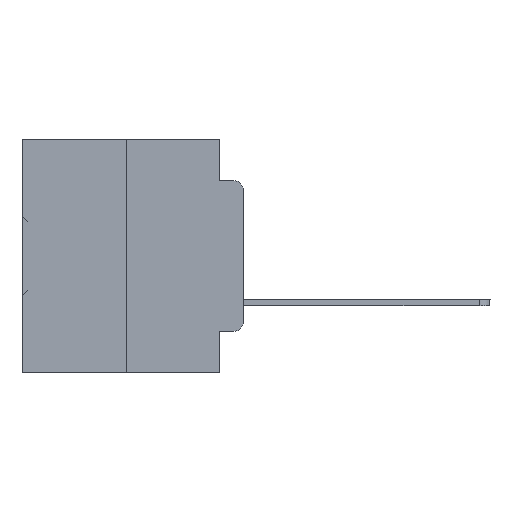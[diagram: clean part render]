
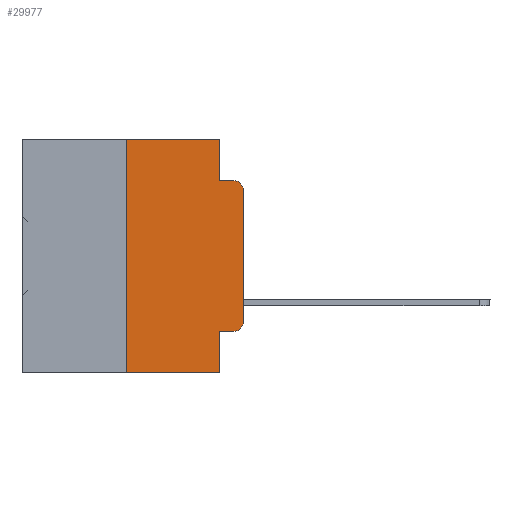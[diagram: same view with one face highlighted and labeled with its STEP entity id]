
A CAD part, left-side view. The second image highlights one B-rep face of the part: STEP entity #29977.
In plain terms, the highlighted planar face has unit normal (-1, 0, 0).
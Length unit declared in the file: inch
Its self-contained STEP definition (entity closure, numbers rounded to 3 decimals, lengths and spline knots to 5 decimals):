
#377 = VERTEX_POINT ( 'NONE', #6065 ) ;
#1059 = AXIS2_PLACEMENT_3D ( 'NONE', #21264, #10166, #18961 ) ;
#1066 = VECTOR ( 'NONE', #21905, 39.37008 ) ;
#1268 = EDGE_CURVE ( 'NONE', #36753, #8072, #4302, .T. ) ;
#1319 = CIRCLE ( 'NONE', #37366, 0.02 ) ;
#1784 = EDGE_CURVE ( 'NONE', #7292, #15828, #33051, .T. ) ;
#2065 = ORIENTED_EDGE ( 'NONE', *, *, #7020, .F. ) ;
#2233 = CARTESIAN_POINT ( 'NONE',  ( 0., 0.051, -0.4115 ) ) ;
#2725 = CARTESIAN_POINT ( 'NONE',  ( 0., 0.051, -0.0885 ) ) ;
#3130 = DIRECTION ( 'NONE',  ( 0., 0., -1. ) ) ;
#4041 = PLANE ( 'NONE',  #1059 ) ;
#4302 = CIRCLE ( 'NONE', #25704, 0.02 ) ;
#4329 = LINE ( 'NONE', #15992, #6823 ) ;
#5412 = LINE ( 'NONE', #23041, #20232 ) ;
#5631 = DIRECTION ( 'NONE',  ( 0., -1., 0. ) ) ;
#5685 = ORIENTED_EDGE ( 'NONE', *, *, #1268, .T. ) ;
#6065 = CARTESIAN_POINT ( 'NONE',  ( 0., 0.051, 0. ) ) ;
#6823 = VECTOR ( 'NONE', #10818, 39.37008 ) ;
#7020 = EDGE_CURVE ( 'NONE', #377, #24045, #9507, .T. ) ;
#7292 = VERTEX_POINT ( 'NONE', #33897 ) ;
#8072 = VERTEX_POINT ( 'NONE', #25919 ) ;
#8078 = EDGE_CURVE ( 'NONE', #24045, #33711, #5412, .T. ) ;
#8488 = EDGE_CURVE ( 'NONE', #22824, #33711, #1319, .T. ) ;
#9168 = CARTESIAN_POINT ( 'NONE',  ( 0., 0.02, -0.3915 ) ) ;
#9328 = VECTOR ( 'NONE', #11818, 39.37008 ) ;
#9507 = LINE ( 'NONE', #24459, #19050 ) ;
#10166 = DIRECTION ( 'NONE',  ( 1., 0., 0. ) ) ;
#10615 = VERTEX_POINT ( 'NONE', #2233 ) ;
#10782 = LINE ( 'NONE', #36632, #1066 ) ;
#10818 = DIRECTION ( 'NONE',  ( 0., 0., 1. ) ) ;
#11084 = ORIENTED_EDGE ( 'NONE', *, *, #30367, .T. ) ;
#11769 = LINE ( 'NONE', #14824, #12660 ) ;
#11818 = DIRECTION ( 'NONE',  ( 0., -1., 0. ) ) ;
#12660 = VECTOR ( 'NONE', #5631, 39.37008 ) ;
#13003 = CARTESIAN_POINT ( 'NONE',  ( 0., 0.02, -0.4115 ) ) ;
#14824 = CARTESIAN_POINT ( 'NONE',  ( 0., 0.473, -0.5 ) ) ;
#14931 = EDGE_CURVE ( 'NONE', #7292, #27083, #11769, .T. ) ;
#15024 = VECTOR ( 'NONE', #16014, 39.37008 ) ;
#15260 = DIRECTION ( 'NONE',  ( 0., 0., -1. ) ) ;
#15752 = EDGE_CURVE ( 'NONE', #15828, #377, #10782, .T. ) ;
#15828 = VERTEX_POINT ( 'NONE', #37564 ) ;
#15992 = CARTESIAN_POINT ( 'NONE',  ( 0., 0., 0. ) ) ;
#16014 = DIRECTION ( 'NONE',  ( 0., 0., 1. ) ) ;
#16962 = ORIENTED_EDGE ( 'NONE', *, *, #8078, .F. ) ;
#17296 = LINE ( 'NONE', #26316, #24579 ) ;
#17748 = ORIENTED_EDGE ( 'NONE', *, *, #15752, .F. ) ;
#18961 = DIRECTION ( 'NONE',  ( 0., 0., -1. ) ) ;
#19050 = VECTOR ( 'NONE', #15260, 39.37008 ) ;
#19583 = DIRECTION ( 'NONE',  ( 0., -1., 0. ) ) ;
#20232 = VECTOR ( 'NONE', #19583, 39.37008 ) ;
#20850 = DIRECTION ( 'NONE',  ( -1., 0., 0. ) ) ;
#21264 = CARTESIAN_POINT ( 'NONE',  ( 0., 0.473, 0. ) ) ;
#21905 = DIRECTION ( 'NONE',  ( 0., -1., 0. ) ) ;
#22824 = VERTEX_POINT ( 'NONE', #26261 ) ;
#23041 = CARTESIAN_POINT ( 'NONE',  ( 0., 0.051, -0.0885 ) ) ;
#24045 = VERTEX_POINT ( 'NONE', #2725 ) ;
#24459 = CARTESIAN_POINT ( 'NONE',  ( 0., 0.051, 0. ) ) ;
#24579 = VECTOR ( 'NONE', #3130, 39.37008 ) ;
#24679 = ORIENTED_EDGE ( 'NONE', *, *, #1784, .F. ) ;
#25392 = ORIENTED_EDGE ( 'NONE', *, *, #8488, .T. ) ;
#25704 = AXIS2_PLACEMENT_3D ( 'NONE', #9168, #20850, #29312 ) ;
#25919 = CARTESIAN_POINT ( 'NONE',  ( 0., 0., -0.3915 ) ) ;
#26261 = CARTESIAN_POINT ( 'NONE',  ( 0., 0., -0.1085 ) ) ;
#26316 = CARTESIAN_POINT ( 'NONE',  ( 0., 0.051, 0. ) ) ;
#26453 = CARTESIAN_POINT ( 'NONE',  ( 0., 0.051, -0.5 ) ) ;
#26750 = LINE ( 'NONE', #32294, #9328 ) ;
#27083 = VERTEX_POINT ( 'NONE', #26453 ) ;
#28027 = CARTESIAN_POINT ( 'NONE',  ( 0., 0.02, -0.0885 ) ) ;
#29312 = DIRECTION ( 'NONE',  ( 0., 0., -1. ) ) ;
#29842 = ORIENTED_EDGE ( 'NONE', *, *, #32867, .T. ) ;
#29977 = ADVANCED_FACE ( 'NONE', ( #30471 ), #4041, .F. ) ;
#30082 = ORIENTED_EDGE ( 'NONE', *, *, #14931, .T. ) ;
#30367 = EDGE_CURVE ( 'NONE', #8072, #22824, #4329, .T. ) ;
#30471 = FACE_OUTER_BOUND ( 'NONE', #30561, .T. ) ;
#30561 = EDGE_LOOP ( 'NONE', ( #11084, #25392, #16962, #2065, #17748, #24679, #30082, #34564, #29842, #5685 ) ) ;
#31418 = DIRECTION ( 'NONE',  ( 0., 0., -1. ) ) ;
#31614 = DIRECTION ( 'NONE',  ( -1., 0., 0. ) ) ;
#32040 = EDGE_CURVE ( 'NONE', #10615, #27083, #17296, .T. ) ;
#32294 = CARTESIAN_POINT ( 'NONE',  ( 0., 0.051, -0.4115 ) ) ;
#32867 = EDGE_CURVE ( 'NONE', #10615, #36753, #26750, .T. ) ;
#32871 = CARTESIAN_POINT ( 'NONE',  ( 0., 0.25, 0. ) ) ;
#33051 = LINE ( 'NONE', #32871, #15024 ) ;
#33711 = VERTEX_POINT ( 'NONE', #28027 ) ;
#33897 = CARTESIAN_POINT ( 'NONE',  ( 0., 0.25, -0.5 ) ) ;
#34564 = ORIENTED_EDGE ( 'NONE', *, *, #32040, .F. ) ;
#36632 = CARTESIAN_POINT ( 'NONE',  ( 0., 0.473, 0. ) ) ;
#36753 = VERTEX_POINT ( 'NONE', #13003 ) ;
#37366 = AXIS2_PLACEMENT_3D ( 'NONE', #37529, #31614, #31418 ) ;
#37529 = CARTESIAN_POINT ( 'NONE',  ( 0., 0.02, -0.1085 ) ) ;
#37564 = CARTESIAN_POINT ( 'NONE',  ( 0., 0.25, 0. ) ) ;
